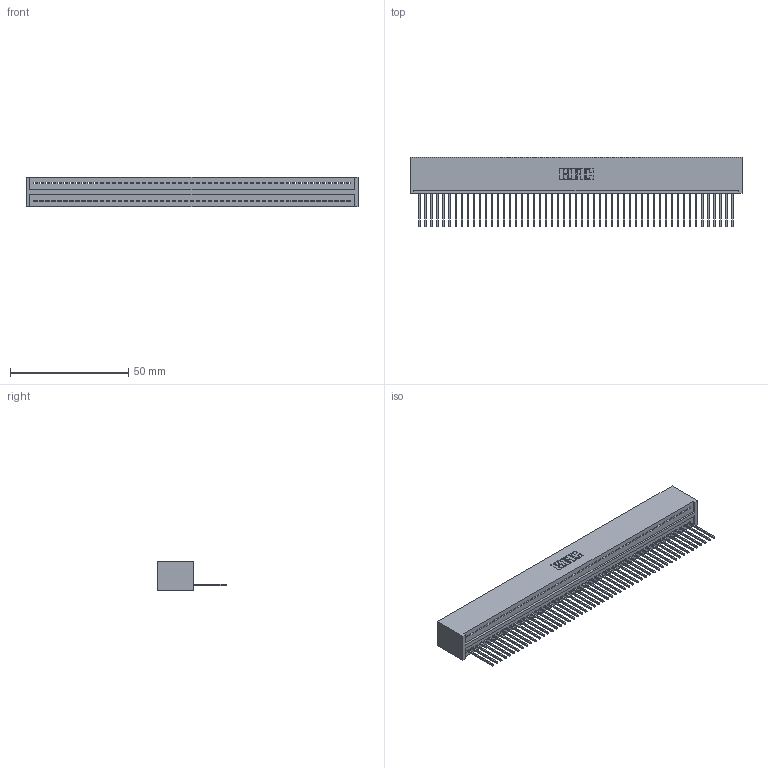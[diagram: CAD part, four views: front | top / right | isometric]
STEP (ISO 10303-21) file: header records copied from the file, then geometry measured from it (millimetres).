
FILE_DESCRIPTION (( 'STEP AP203' ), '1' );
FILE_NAME ('325-053-540-101.STEP', '2020-02-25T00:42:06', ( '' ), ( '' ), 'SwSTEP 2.0', 'SolidWorks 2016', '' );
FILE_SCHEMA (( 'CONFIG_CONTROL_DESIGN' ));
Length unit declared in the file: inch
Products named in the file (3): 325-292-001_325-293-140; 325 Part_Lugless; 325-053-540-101
Assembly tree (54 placements, depth 2):
  325-053-540-101
    325 Part_Lugless
    325-292-001_325-293-140  x53
Bounding box: 140.26 x 29.46 x 12.45 mm (x, y, z)
Volume: 18536 mm3; surface area: 21458.5 mm2
Topology: 54 solids, 54 shells, 3180 faces, 9615 edges, 6338 vertices
Faces by surface type: plane 2292, cylinder 888
Entity records: 30719 total; most frequent: CARTESIAN_POINT 5305, ORIENTED_EDGE 5294, DIRECTION 4445, EDGE_CURVE 2647, LINE 2527, VECTOR 2527, VERTEX_POINT 1762, AXIS2_PLACEMENT_3D 959
